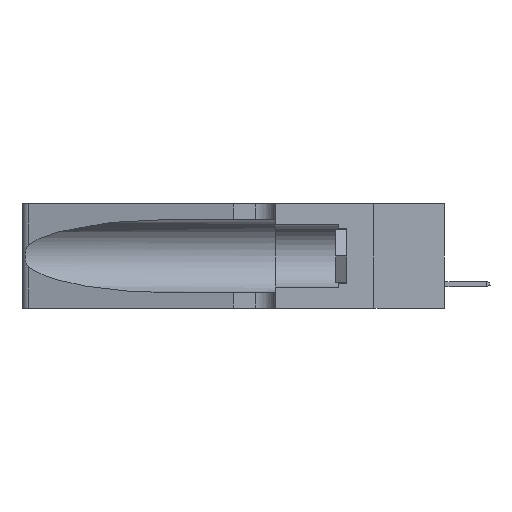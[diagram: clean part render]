
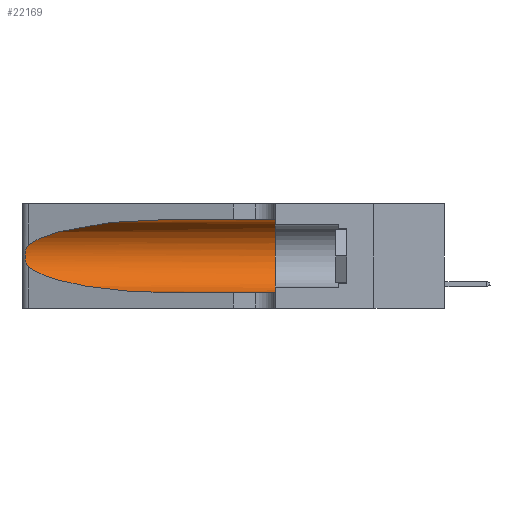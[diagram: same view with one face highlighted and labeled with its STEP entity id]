
A CAD part, left-side view. The second image highlights one B-rep face of the part: STEP entity #22169.
In plain terms, the highlighted cylindrical face has radius 3.308 mm (diameter 6.617 mm), a partial arc.
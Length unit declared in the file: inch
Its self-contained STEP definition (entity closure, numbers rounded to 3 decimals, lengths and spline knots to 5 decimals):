
#2096 = CARTESIAN_POINT ( 'NONE',  ( 0.25555, 1.22994, 0.2215 ) ) ;
#2275 = CARTESIAN_POINT ( 'NONE',  ( 0.25854, 1.2359, 0.20912 ) ) ;
#2990 = CARTESIAN_POINT ( 'NONE',  ( 0.1305, 0.35, 0.31525 ) ) ;
#6178 = CARTESIAN_POINT ( 'NONE',  ( 0.26075, 1.23896, 0.178 ) ) ;
#6562 = ORIENTED_EDGE ( 'NONE', *, *, #25177, .F. ) ;
#6695 = CARTESIAN_POINT ( 'NONE',  ( 0.25787, 1.23484, 0.2124 ) ) ;
#8029 =( BOUNDED_CURVE ( )  B_SPLINE_CURVE ( 3, ( #25107, #29331, #33572, #41147 ),
 .UNSPECIFIED., .F., .F. ) 
 B_SPLINE_CURVE_WITH_KNOTS ( ( 4, 4 ),
 ( 1.5708, 2.84003 ),
 .UNSPECIFIED. ) 
 CURVE ( )  GEOMETRIC_REPRESENTATION_ITEM ( )  RATIONAL_B_SPLINE_CURVE ( ( 1., 0.87, 0.87, 1. ) ) 
 REPRESENTATION_ITEM ( '' )  );
#8204 = VERTEX_POINT ( 'NONE', #40166 ) ;
#8796 = CARTESIAN_POINT ( 'NONE',  ( 0.1305, 0.72297, 0.05475 ) ) ;
#10045 = CARTESIAN_POINT ( 'NONE',  ( 0.26018, 1.23835, 0.19895 ) ) ;
#10726 = CARTESIAN_POINT ( 'NONE',  ( 0.25789, 1.23486, 0.15765 ) ) ;
#10771 = LINE ( 'NONE', #23460, #51226 ) ;
#12245 = EDGE_CURVE ( 'NONE', #47362, #35568, #25540, .T. ) ;
#14704 = VERTEX_POINT ( 'NONE', #15155 ) ;
#14801 = EDGE_LOOP ( 'NONE', ( #40316, #46332, #37897, #29542, #34332, #6562 ) ) ;
#14808 = CARTESIAN_POINT ( 'NONE',  ( 0.25639, 1.23186, 0.15144 ) ) ;
#14912 = CYLINDRICAL_SURFACE ( 'NONE', #16923, 0.13025 ) ;
#15155 = CARTESIAN_POINT ( 'NONE',  ( 0.25487, 1.22718, 0.22369 ) ) ;
#15631 = CARTESIAN_POINT ( 'NONE',  ( 0.1305, 0.35, 0.05475 ) ) ;
#16923 = AXIS2_PLACEMENT_3D ( 'NONE', #21840, #25578, #33682 ) ;
#17310 = EDGE_CURVE ( 'NONE', #39527, #47362, #44605, .T. ) ;
#17421 = FACE_OUTER_BOUND ( 'NONE', #14801, .T. ) ;
#18324 = CARTESIAN_POINT ( 'NONE',  ( 0.25487, 1.22718, 0.14631 ) ) ;
#19202 = CARTESIAN_POINT ( 'NONE',  ( 0.1305, 1.61858, 0.05475 ) ) ;
#21642 = EDGE_CURVE ( 'NONE', #14704, #39527, #39070, .T. ) ;
#21840 = CARTESIAN_POINT ( 'NONE',  ( 0.1305, 1.61858, 0.185 ) ) ;
#21916 = EDGE_CURVE ( 'NONE', #31216, #35568, #38326, .T. ) ;
#22169 = ADVANCED_FACE ( 'NONE', ( #17421 ), #14912, .F. ) ;
#23460 = CARTESIAN_POINT ( 'NONE',  ( 0.1305, 1.61858, 0.31525 ) ) ;
#23997 = DIRECTION ( 'NONE',  ( 0., 1., 0. ) ) ;
#24720 = EDGE_CURVE ( 'NONE', #8204, #14704, #8029, .T. ) ;
#25107 = CARTESIAN_POINT ( 'NONE',  ( 0.1305, 0.72297, 0.31525 ) ) ;
#25177 = EDGE_CURVE ( 'NONE', #8204, #31216, #10771, .T. ) ;
#25540 = LINE ( 'NONE', #19202, #28059 ) ;
#25578 = DIRECTION ( 'NONE',  ( 0., -1., 0. ) ) ;
#26980 = CARTESIAN_POINT ( 'NONE',  ( 0.1305, 0.72297, 0.05475 ) ) ;
#28059 = VECTOR ( 'NONE', #39543, 39.37008 ) ;
#29331 = CARTESIAN_POINT ( 'NONE',  ( 0.18966, 0.96281, 0.31525 ) ) ;
#29542 = ORIENTED_EDGE ( 'NONE', *, *, #12245, .T. ) ;
#31216 = VERTEX_POINT ( 'NONE', #2990 ) ;
#33572 = CARTESIAN_POINT ( 'NONE',  ( 0.2373, 1.15595, 0.28018 ) ) ;
#33682 = DIRECTION ( 'NONE',  ( 0., 0., -1. ) ) ;
#34332 = ORIENTED_EDGE ( 'NONE', *, *, #21916, .F. ) ;
#34902 = CARTESIAN_POINT ( 'NONE',  ( 0.25487, 1.22718, 0.14631 ) ) ;
#34939 = CARTESIAN_POINT ( 'NONE',  ( 0.25856, 1.23593, 0.16098 ) ) ;
#35568 = VERTEX_POINT ( 'NONE', #15631 ) ;
#36003 = DIRECTION ( 'NONE',  ( 0., 0., 1. ) ) ;
#37897 = ORIENTED_EDGE ( 'NONE', *, *, #17310, .T. ) ;
#38326 = CIRCLE ( 'NONE', #50453, 0.13025 ) ;
#38473 = CARTESIAN_POINT ( 'NONE',  ( 0.25555, 1.22993, 0.14849 ) ) ;
#38801 = CARTESIAN_POINT ( 'NONE',  ( 0.26017, 1.23833, 0.17102 ) ) ;
#38986 = CARTESIAN_POINT ( 'NONE',  ( 0.25639, 1.23184, 0.21858 ) ) ;
#39070 = B_SPLINE_CURVE_WITH_KNOTS ( 'NONE', 3,
 ( #50487, #2096, #38986, #6695, #2275, #10045, #46921, #6178, #38801, #34939, #10726, #14808, #38473, #18324 ),
 .UNSPECIFIED., .F., .F.,
 ( 4, 2, 2, 2, 2, 2, 4 ),
 ( 0., 0.00027, 0.00053, 0.00107, 0.0016, 0.00187, 0.00214 ),
 .UNSPECIFIED. ) ;
#39527 = VERTEX_POINT ( 'NONE', #41331 ) ;
#39543 = DIRECTION ( 'NONE',  ( 0., -1., 0. ) ) ;
#40166 = CARTESIAN_POINT ( 'NONE',  ( 0.1305, 0.72297, 0.31525 ) ) ;
#40316 = ORIENTED_EDGE ( 'NONE', *, *, #24720, .T. ) ;
#41147 = CARTESIAN_POINT ( 'NONE',  ( 0.25487, 1.22718, 0.22369 ) ) ;
#41331 = CARTESIAN_POINT ( 'NONE',  ( 0.25487, 1.22718, 0.14631 ) ) ;
#44292 = CARTESIAN_POINT ( 'NONE',  ( 0.1305, 0.35, 0.185 ) ) ;
#44605 =( BOUNDED_CURVE ( )  B_SPLINE_CURVE ( 3, ( #34902, #51859, #51690, #26980 ),
 .UNSPECIFIED., .F., .F. ) 
 B_SPLINE_CURVE_WITH_KNOTS ( ( 4, 4 ),
 ( 3.44316, 4.71239 ),
 .UNSPECIFIED. ) 
 CURVE ( )  GEOMETRIC_REPRESENTATION_ITEM ( )  RATIONAL_B_SPLINE_CURVE ( ( 1., 0.87, 0.87, 1. ) ) 
 REPRESENTATION_ITEM ( '' )  );
#46332 = ORIENTED_EDGE ( 'NONE', *, *, #21642, .T. ) ;
#46921 = CARTESIAN_POINT ( 'NONE',  ( 0.26075, 1.23896, 0.19203 ) ) ;
#47362 = VERTEX_POINT ( 'NONE', #8796 ) ;
#50453 = AXIS2_PLACEMENT_3D ( 'NONE', #44292, #23997, #36003 ) ;
#50487 = CARTESIAN_POINT ( 'NONE',  ( 0.25487, 1.22718, 0.22369 ) ) ;
#51226 = VECTOR ( 'NONE', #51903, 39.37008 ) ;
#51690 = CARTESIAN_POINT ( 'NONE',  ( 0.18966, 0.96281, 0.05475 ) ) ;
#51859 = CARTESIAN_POINT ( 'NONE',  ( 0.2373, 1.15595, 0.08982 ) ) ;
#51903 = DIRECTION ( 'NONE',  ( 0., -1., 0. ) ) ;
